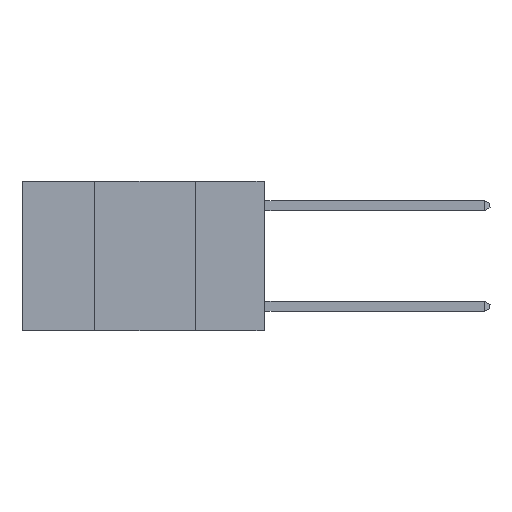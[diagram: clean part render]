
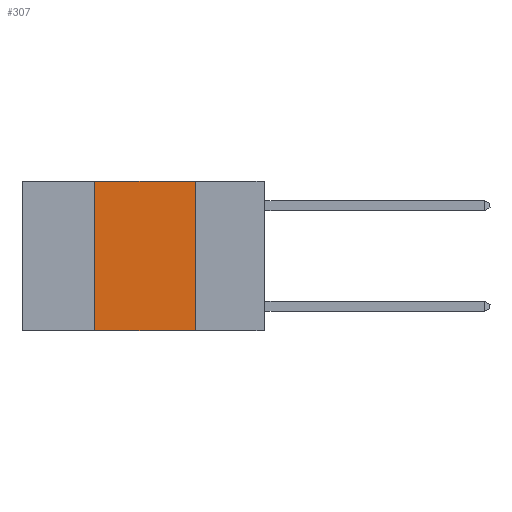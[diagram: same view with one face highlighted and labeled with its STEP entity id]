
A CAD part, left-side view. The second image highlights one B-rep face of the part: STEP entity #307.
In plain terms, the highlighted planar face has unit normal (-1, 0, 0).
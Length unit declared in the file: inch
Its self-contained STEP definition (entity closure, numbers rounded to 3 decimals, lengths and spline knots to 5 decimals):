
#68 = EDGE_CURVE ( 'NONE', #6335, #6527, #9467, .T. ) ;
#117 = AXIS2_PLACEMENT_3D ( 'NONE', #3657, #4573, #4407 ) ;
#307 = ADVANCED_FACE ( 'NONE', ( #7328 ), #9745, .F. ) ;
#453 = LINE ( 'NONE', #875, #6408 ) ;
#875 = CARTESIAN_POINT ( 'NONE',  ( 0., 0.6, -0.37 ) ) ;
#1492 = VECTOR ( 'NONE', #9031, 39.37008 ) ;
#1690 = DIRECTION ( 'NONE',  ( 0., -1., 0. ) ) ;
#1863 = CARTESIAN_POINT ( 'NONE',  ( 0., 0.42, 0. ) ) ;
#1903 = ORIENTED_EDGE ( 'NONE', *, *, #3305, .T. ) ;
#2407 = DIRECTION ( 'NONE',  ( 0., -1., 0. ) ) ;
#2651 = CARTESIAN_POINT ( 'NONE',  ( 0., 0.17, -0.37 ) ) ;
#3191 = VERTEX_POINT ( 'NONE', #7506 ) ;
#3247 = VECTOR ( 'NONE', #1690, 39.37008 ) ;
#3305 = EDGE_CURVE ( 'NONE', #6335, #8142, #453, .T. ) ;
#3657 = CARTESIAN_POINT ( 'NONE',  ( 0., 0.6, 0. ) ) ;
#4407 = DIRECTION ( 'NONE',  ( 0., 0., -1. ) ) ;
#4573 = DIRECTION ( 'NONE',  ( 1., 0., 0. ) ) ;
#5223 = ORIENTED_EDGE ( 'NONE', *, *, #6360, .F. ) ;
#5587 = ORIENTED_EDGE ( 'NONE', *, *, #9020, .F. ) ;
#6335 = VERTEX_POINT ( 'NONE', #7124 ) ;
#6360 = EDGE_CURVE ( 'NONE', #6527, #3191, #7397, .T. ) ;
#6408 = VECTOR ( 'NONE', #2407, 39.37008 ) ;
#6527 = VERTEX_POINT ( 'NONE', #1863 ) ;
#7124 = CARTESIAN_POINT ( 'NONE',  ( 0., 0.42, -0.37 ) ) ;
#7328 = FACE_OUTER_BOUND ( 'NONE', #9881, .T. ) ;
#7397 = LINE ( 'NONE', #9411, #3247 ) ;
#7506 = CARTESIAN_POINT ( 'NONE',  ( 0., 0.17, 0. ) ) ;
#7704 = VECTOR ( 'NONE', #9073, 39.37008 ) ;
#7774 = ORIENTED_EDGE ( 'NONE', *, *, #68, .F. ) ;
#8142 = VERTEX_POINT ( 'NONE', #2651 ) ;
#8278 = CARTESIAN_POINT ( 'NONE',  ( 0., 0.17, 0. ) ) ;
#9020 = EDGE_CURVE ( 'NONE', #3191, #8142, #9716, .T. ) ;
#9031 = DIRECTION ( 'NONE',  ( 0., 0., -1. ) ) ;
#9073 = DIRECTION ( 'NONE',  ( 0., 0., 1. ) ) ;
#9411 = CARTESIAN_POINT ( 'NONE',  ( 0., 0.6, 0. ) ) ;
#9467 = LINE ( 'NONE', #9504, #7704 ) ;
#9504 = CARTESIAN_POINT ( 'NONE',  ( 0., 0.42, 0. ) ) ;
#9716 = LINE ( 'NONE', #8278, #1492 ) ;
#9745 = PLANE ( 'NONE',  #117 ) ;
#9881 = EDGE_LOOP ( 'NONE', ( #5587, #5223, #7774, #1903 ) ) ;
